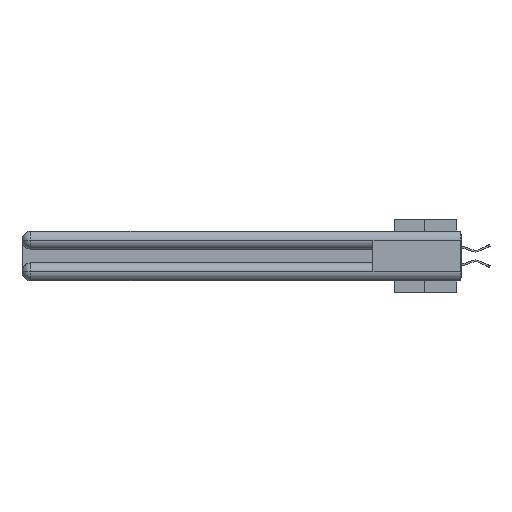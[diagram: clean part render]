
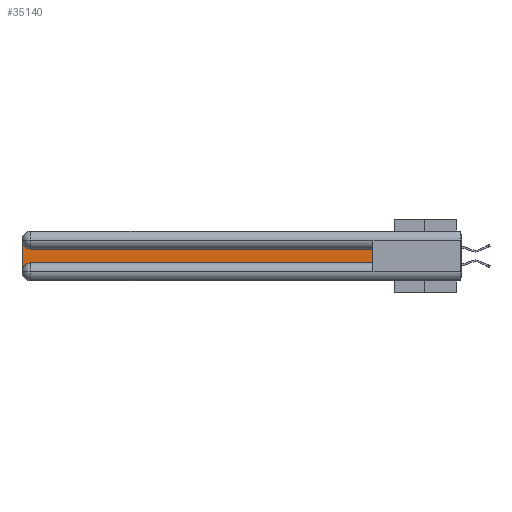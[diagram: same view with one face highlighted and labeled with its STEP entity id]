
A CAD part, left-side view. The second image highlights one B-rep face of the part: STEP entity #35140.
In plain terms, the highlighted planar face has unit normal (-1, 0, 0).
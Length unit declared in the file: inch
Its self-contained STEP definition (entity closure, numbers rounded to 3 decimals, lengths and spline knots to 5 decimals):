
#774 = CARTESIAN_POINT ( 'NONE',  ( 0.075, 0.6, -0.2175 ) ) ;
#1352 = CARTESIAN_POINT ( 'NONE',  ( 0.075, 2.94, -0.2775 ) ) ;
#4462 = CIRCLE ( 'NONE', #33516, 0.06 ) ;
#5168 = DIRECTION ( 'NONE',  ( 0., 0., -1. ) ) ;
#5210 = CARTESIAN_POINT ( 'NONE',  ( 0.075, 2.94, -0.0625 ) ) ;
#5401 = VERTEX_POINT ( 'NONE', #33093 ) ;
#6690 = CARTESIAN_POINT ( 'NONE',  ( 0.075, 3., -0.1225 ) ) ;
#6859 = DIRECTION ( 'NONE',  ( 0., -1., 0. ) ) ;
#7006 = LINE ( 'NONE', #28165, #29974 ) ;
#8533 = VERTEX_POINT ( 'NONE', #23913 ) ;
#8896 = ORIENTED_EDGE ( 'NONE', *, *, #38474, .T. ) ;
#9674 = CARTESIAN_POINT ( 'NONE',  ( 0.075, 3., -0.2775 ) ) ;
#9706 = EDGE_CURVE ( 'NONE', #28702, #25885, #23992, .T. ) ;
#9708 = AXIS2_PLACEMENT_3D ( 'NONE', #5210, #26649, #20129 ) ;
#10565 = FACE_OUTER_BOUND ( 'NONE', #32218, .T. ) ;
#10908 = EDGE_CURVE ( 'NONE', #26142, #8533, #31175, .T. ) ;
#12015 = VECTOR ( 'NONE', #20434, 39.37008 ) ;
#12311 = PLANE ( 'NONE',  #22952 ) ;
#13493 = CARTESIAN_POINT ( 'NONE',  ( 0.075, 0.6, -0.1225 ) ) ;
#16245 = LINE ( 'NONE', #39206, #25339 ) ;
#16474 = VERTEX_POINT ( 'NONE', #9674 ) ;
#18388 = CARTESIAN_POINT ( 'NONE',  ( 0.075, 0.6, -0.2175 ) ) ;
#18580 = CARTESIAN_POINT ( 'NONE',  ( 0.075, 2.94, -0.2175 ) ) ;
#20129 = DIRECTION ( 'NONE',  ( 0., 0., -1. ) ) ;
#20434 = DIRECTION ( 'NONE',  ( 0., 1., 0. ) ) ;
#21819 = DIRECTION ( 'NONE',  ( 0., 0., -1. ) ) ;
#21900 = ORIENTED_EDGE ( 'NONE', *, *, #31531, .T. ) ;
#22952 = AXIS2_PLACEMENT_3D ( 'NONE', #6690, #30751, #21819 ) ;
#23913 = CARTESIAN_POINT ( 'NONE',  ( 0.075, 2.94, -0.1225 ) ) ;
#23992 = LINE ( 'NONE', #18388, #28809 ) ;
#24203 = EDGE_CURVE ( 'NONE', #25885, #26142, #7006, .T. ) ;
#25339 = VECTOR ( 'NONE', #5168, 39.37008 ) ;
#25844 = DIRECTION ( 'NONE',  ( 0., 0., -1. ) ) ;
#25885 = VERTEX_POINT ( 'NONE', #774 ) ;
#26137 = ORIENTED_EDGE ( 'NONE', *, *, #30346, .T. ) ;
#26142 = VERTEX_POINT ( 'NONE', #30428 ) ;
#26649 = DIRECTION ( 'NONE',  ( 1., 0., 0. ) ) ;
#28165 = CARTESIAN_POINT ( 'NONE',  ( 0.075, 0.6, -0.2175 ) ) ;
#28702 = VERTEX_POINT ( 'NONE', #18580 ) ;
#28809 = VECTOR ( 'NONE', #6859, 39.37008 ) ;
#29765 = ORIENTED_EDGE ( 'NONE', *, *, #24203, .T. ) ;
#29974 = VECTOR ( 'NONE', #37280, 39.37008 ) ;
#30346 = EDGE_CURVE ( 'NONE', #5401, #16474, #16245, .T. ) ;
#30428 = CARTESIAN_POINT ( 'NONE',  ( 0.075, 0.6, -0.1225 ) ) ;
#30751 = DIRECTION ( 'NONE',  ( 1., 0., 0. ) ) ;
#31175 = LINE ( 'NONE', #13493, #12015 ) ;
#31479 = CIRCLE ( 'NONE', #9708, 0.06 ) ;
#31531 = EDGE_CURVE ( 'NONE', #8533, #5401, #31479, .T. ) ;
#32218 = EDGE_LOOP ( 'NONE', ( #35525, #21900, #26137, #8896, #38829, #29765 ) ) ;
#33093 = CARTESIAN_POINT ( 'NONE',  ( 0.075, 3., -0.0625 ) ) ;
#33516 = AXIS2_PLACEMENT_3D ( 'NONE', #1352, #35349, #25844 ) ;
#35140 = ADVANCED_FACE ( 'NONE', ( #10565 ), #12311, .F. ) ;
#35349 = DIRECTION ( 'NONE',  ( 1., 0., 0. ) ) ;
#35525 = ORIENTED_EDGE ( 'NONE', *, *, #10908, .T. ) ;
#37280 = DIRECTION ( 'NONE',  ( 0., 0., 1. ) ) ;
#38474 = EDGE_CURVE ( 'NONE', #16474, #28702, #4462, .T. ) ;
#38829 = ORIENTED_EDGE ( 'NONE', *, *, #9706, .T. ) ;
#39206 = CARTESIAN_POINT ( 'NONE',  ( 0.075, 3., -0.2175 ) ) ;
